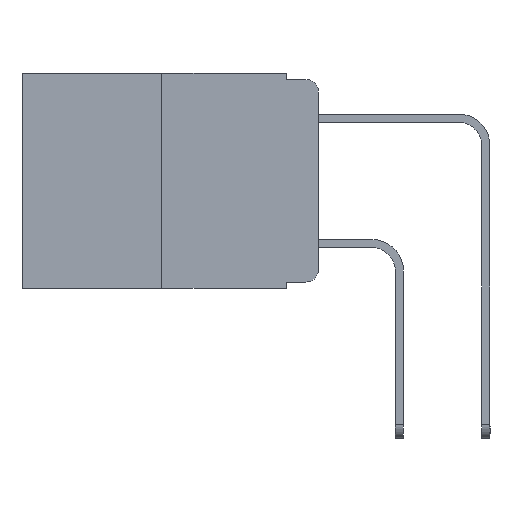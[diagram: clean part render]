
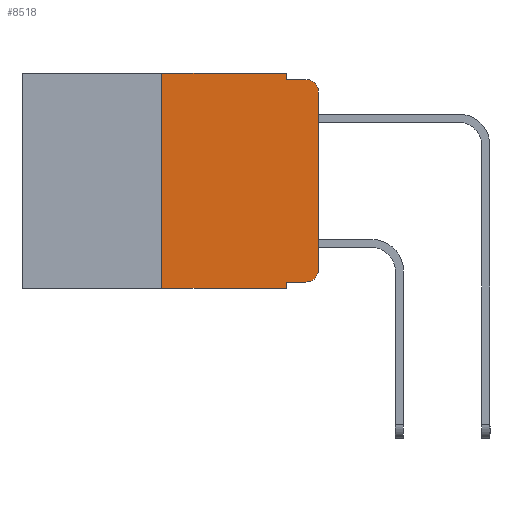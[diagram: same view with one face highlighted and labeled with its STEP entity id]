
A CAD part, left-side view. The second image highlights one B-rep face of the part: STEP entity #8518.
In plain terms, the highlighted planar face has unit normal (-1, 0, 0).
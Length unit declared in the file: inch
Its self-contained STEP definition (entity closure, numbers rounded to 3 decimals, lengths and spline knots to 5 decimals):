
#169 = EDGE_CURVE ( 'NONE', #13300, #1268, #2343, .T. ) ;
#176 = VERTEX_POINT ( 'NONE', #12174 ) ;
#186 = LINE ( 'NONE', #1338, #10568 ) ;
#308 = VECTOR ( 'NONE', #12533, 39.37008 ) ;
#378 = LINE ( 'NONE', #12783, #6785 ) ;
#436 = DIRECTION ( 'NONE',  ( 0., -1., 0. ) ) ;
#512 = AXIS2_PLACEMENT_3D ( 'NONE', #3427, #1086, #12291 ) ;
#872 = EDGE_CURVE ( 'NONE', #4846, #10236, #4366, .T. ) ;
#897 = CARTESIAN_POINT ( 'NONE',  ( 0., 0.473, -0.343 ) ) ;
#941 = CARTESIAN_POINT ( 'NONE',  ( 0., 0.02, -0.03 ) ) ;
#1086 = DIRECTION ( 'NONE',  ( -1., 0., 0. ) ) ;
#1133 = ORIENTED_EDGE ( 'NONE', *, *, #8077, .T. ) ;
#1142 = CARTESIAN_POINT ( 'NONE',  ( 0., 0.25, 0. ) ) ;
#1268 = VERTEX_POINT ( 'NONE', #1142 ) ;
#1338 = CARTESIAN_POINT ( 'NONE',  ( 0., 0., 0. ) ) ;
#1571 = LINE ( 'NONE', #6231, #7298 ) ;
#1618 = VERTEX_POINT ( 'NONE', #4338 ) ;
#2343 = LINE ( 'NONE', #11216, #5552 ) ;
#2546 = EDGE_CURVE ( 'NONE', #4061, #176, #10858, .T. ) ;
#2570 = EDGE_CURVE ( 'NONE', #5635, #4846, #186, .T. ) ;
#2621 = CARTESIAN_POINT ( 'NONE',  ( 0., 0.02, -0.333 ) ) ;
#2679 = ORIENTED_EDGE ( 'NONE', *, *, #169, .F. ) ;
#2816 = VECTOR ( 'NONE', #8243, 39.37008 ) ;
#2945 = CARTESIAN_POINT ( 'NONE',  ( 0., 0.473, 0. ) ) ;
#3021 = DIRECTION ( 'NONE',  ( 0., -1., 0. ) ) ;
#3113 = ORIENTED_EDGE ( 'NONE', *, *, #2570, .T. ) ;
#3191 = EDGE_LOOP ( 'NONE', ( #3113, #8809, #12983, #13635, #10207, #2679, #1133, #9418, #4559, #13955 ) ) ;
#3427 = CARTESIAN_POINT ( 'NONE',  ( 0., 0.02, -0.313 ) ) ;
#3856 = CARTESIAN_POINT ( 'NONE',  ( 0., 0.02, -0.01 ) ) ;
#3927 = CARTESIAN_POINT ( 'NONE',  ( 0., 0.051, 0. ) ) ;
#4009 = PLANE ( 'NONE',  #5604 ) ;
#4061 = VERTEX_POINT ( 'NONE', #6833 ) ;
#4338 = CARTESIAN_POINT ( 'NONE',  ( 0., 0.051, -0.01 ) ) ;
#4366 = CIRCLE ( 'NONE', #10379, 0.02 ) ;
#4559 = ORIENTED_EDGE ( 'NONE', *, *, #10961, .T. ) ;
#4672 = DIRECTION ( 'NONE',  ( 0., 0., 1. ) ) ;
#4782 = DIRECTION ( 'NONE',  ( 0., -1., 0. ) ) ;
#4846 = VERTEX_POINT ( 'NONE', #12142 ) ;
#5107 = CARTESIAN_POINT ( 'NONE',  ( 0., 0.051, 0. ) ) ;
#5416 = CARTESIAN_POINT ( 'NONE',  ( 0., 0., -0.313 ) ) ;
#5552 = VECTOR ( 'NONE', #5727, 39.37008 ) ;
#5604 = AXIS2_PLACEMENT_3D ( 'NONE', #2945, #14146, #10775 ) ;
#5625 = DIRECTION ( 'NONE',  ( -1., 0., 0. ) ) ;
#5635 = VERTEX_POINT ( 'NONE', #5416 ) ;
#5727 = DIRECTION ( 'NONE',  ( 0., 0., 1. ) ) ;
#5859 = CARTESIAN_POINT ( 'NONE',  ( 0., 0.051, 0. ) ) ;
#5882 = CIRCLE ( 'NONE', #512, 0.02 ) ;
#6231 = CARTESIAN_POINT ( 'NONE',  ( 0., 0.473, 0. ) ) ;
#6483 = DIRECTION ( 'NONE',  ( 0., 0., -1. ) ) ;
#6785 = VECTOR ( 'NONE', #436, 39.37008 ) ;
#6833 = CARTESIAN_POINT ( 'NONE',  ( 0., 0.051, -0.333 ) ) ;
#7168 = VERTEX_POINT ( 'NONE', #3927 ) ;
#7298 = VECTOR ( 'NONE', #4782, 39.37008 ) ;
#7437 = VECTOR ( 'NONE', #3021, 39.37008 ) ;
#7654 = FACE_OUTER_BOUND ( 'NONE', #3191, .T. ) ;
#8077 = EDGE_CURVE ( 'NONE', #13300, #176, #12907, .T. ) ;
#8243 = DIRECTION ( 'NONE',  ( 0., 0., -1. ) ) ;
#8518 = ADVANCED_FACE ( 'NONE', ( #7654 ), #4009, .F. ) ;
#8809 = ORIENTED_EDGE ( 'NONE', *, *, #872, .T. ) ;
#9287 = CARTESIAN_POINT ( 'NONE',  ( 0., 0.25, -0.343 ) ) ;
#9418 = ORIENTED_EDGE ( 'NONE', *, *, #2546, .F. ) ;
#9590 = EDGE_CURVE ( 'NONE', #7168, #1618, #12892, .T. ) ;
#10157 = VERTEX_POINT ( 'NONE', #2621 ) ;
#10201 = EDGE_CURVE ( 'NONE', #1618, #10236, #378, .T. ) ;
#10207 = ORIENTED_EDGE ( 'NONE', *, *, #13689, .F. ) ;
#10236 = VERTEX_POINT ( 'NONE', #3856 ) ;
#10338 = DIRECTION ( 'NONE',  ( 0., 0., -1. ) ) ;
#10379 = AXIS2_PLACEMENT_3D ( 'NONE', #941, #5625, #6483 ) ;
#10541 = EDGE_CURVE ( 'NONE', #10157, #5635, #5882, .T. ) ;
#10568 = VECTOR ( 'NONE', #4672, 39.37008 ) ;
#10775 = DIRECTION ( 'NONE',  ( 0., 0., -1. ) ) ;
#10858 = LINE ( 'NONE', #5859, #13110 ) ;
#10961 = EDGE_CURVE ( 'NONE', #4061, #10157, #12477, .T. ) ;
#11216 = CARTESIAN_POINT ( 'NONE',  ( 0., 0.25, 0. ) ) ;
#12142 = CARTESIAN_POINT ( 'NONE',  ( 0., 0., -0.03 ) ) ;
#12174 = CARTESIAN_POINT ( 'NONE',  ( 0., 0.051, -0.343 ) ) ;
#12291 = DIRECTION ( 'NONE',  ( 0., 0., -1. ) ) ;
#12407 = CARTESIAN_POINT ( 'NONE',  ( 0., 0.051, -0.333 ) ) ;
#12477 = LINE ( 'NONE', #12407, #308 ) ;
#12533 = DIRECTION ( 'NONE',  ( 0., -1., 0. ) ) ;
#12783 = CARTESIAN_POINT ( 'NONE',  ( 0., 0.051, -0.01 ) ) ;
#12892 = LINE ( 'NONE', #5107, #2816 ) ;
#12907 = LINE ( 'NONE', #897, #7437 ) ;
#12983 = ORIENTED_EDGE ( 'NONE', *, *, #10201, .F. ) ;
#13110 = VECTOR ( 'NONE', #10338, 39.37008 ) ;
#13300 = VERTEX_POINT ( 'NONE', #9287 ) ;
#13635 = ORIENTED_EDGE ( 'NONE', *, *, #9590, .F. ) ;
#13689 = EDGE_CURVE ( 'NONE', #1268, #7168, #1571, .T. ) ;
#13955 = ORIENTED_EDGE ( 'NONE', *, *, #10541, .T. ) ;
#14146 = DIRECTION ( 'NONE',  ( 1., 0., 0. ) ) ;
